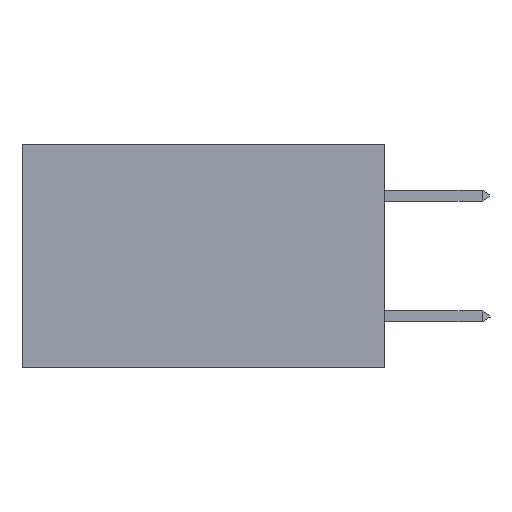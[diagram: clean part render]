
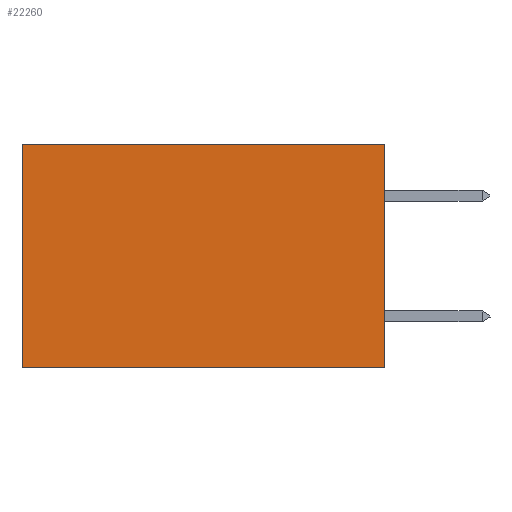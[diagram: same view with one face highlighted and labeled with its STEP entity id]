
A CAD part, left-side view. The second image highlights one B-rep face of the part: STEP entity #22260.
In plain terms, the highlighted planar face has unit normal (-1, 0, 0).
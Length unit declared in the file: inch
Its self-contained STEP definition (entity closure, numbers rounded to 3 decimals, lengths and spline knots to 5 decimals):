
#499 = LINE ( 'NONE', #30578, #22509 ) ;
#1411 = CARTESIAN_POINT ( 'NONE',  ( 0.2875, 0., 0. ) ) ;
#1512 = ORIENTED_EDGE ( 'NONE', *, *, #26970, .F. ) ;
#2909 = CARTESIAN_POINT ( 'NONE',  ( 0.2875, 0., 0. ) ) ;
#3466 = VERTEX_POINT ( 'NONE', #15081 ) ;
#4373 = CARTESIAN_POINT ( 'NONE',  ( 0.2875, 0.6, -0.37 ) ) ;
#5432 = LINE ( 'NONE', #27463, #14908 ) ;
#6847 = EDGE_LOOP ( 'NONE', ( #8869, #7572, #1512, #26331 ) ) ;
#7572 = ORIENTED_EDGE ( 'NONE', *, *, #21735, .F. ) ;
#7997 = VECTOR ( 'NONE', #22997, 39.37008 ) ;
#8869 = ORIENTED_EDGE ( 'NONE', *, *, #30475, .T. ) ;
#10986 = DIRECTION ( 'NONE',  ( 1., 0., 0. ) ) ;
#11207 = CARTESIAN_POINT ( 'NONE',  ( 0.2875, 0.6, 0. ) ) ;
#11342 = DIRECTION ( 'NONE',  ( 0., 0., -1. ) ) ;
#11831 = LINE ( 'NONE', #28019, #7997 ) ;
#14504 = LINE ( 'NONE', #27450, #29020 ) ;
#14908 = VECTOR ( 'NONE', #27703, 39.37008 ) ;
#15081 = CARTESIAN_POINT ( 'NONE',  ( 0.2875, 0., -0.37 ) ) ;
#17165 = FACE_OUTER_BOUND ( 'NONE', #6847, .T. ) ;
#17415 = PLANE ( 'NONE',  #24161 ) ;
#18496 = DIRECTION ( 'NONE',  ( 0., 1., 0. ) ) ;
#18920 = VERTEX_POINT ( 'NONE', #1411 ) ;
#19994 = VERTEX_POINT ( 'NONE', #4373 ) ;
#21735 = EDGE_CURVE ( 'NONE', #3466, #19994, #5432, .T. ) ;
#22260 = ADVANCED_FACE ( 'NONE', ( #17165 ), #17415, .F. ) ;
#22509 = VECTOR ( 'NONE', #11342, 39.37008 ) ;
#22997 = DIRECTION ( 'NONE',  ( 0., 0., -1. ) ) ;
#24161 = AXIS2_PLACEMENT_3D ( 'NONE', #2909, #10986, #30115 ) ;
#24258 = VERTEX_POINT ( 'NONE', #11207 ) ;
#25788 = EDGE_CURVE ( 'NONE', #18920, #24258, #14504, .T. ) ;
#26331 = ORIENTED_EDGE ( 'NONE', *, *, #25788, .T. ) ;
#26970 = EDGE_CURVE ( 'NONE', #18920, #3466, #11831, .T. ) ;
#27450 = CARTESIAN_POINT ( 'NONE',  ( 0.2875, 0., 0. ) ) ;
#27463 = CARTESIAN_POINT ( 'NONE',  ( 0.2875, 0., -0.37 ) ) ;
#27703 = DIRECTION ( 'NONE',  ( 0., 1., 0. ) ) ;
#28019 = CARTESIAN_POINT ( 'NONE',  ( 0.2875, 0., 0. ) ) ;
#29020 = VECTOR ( 'NONE', #18496, 39.37008 ) ;
#30115 = DIRECTION ( 'NONE',  ( 0., 0., -1. ) ) ;
#30475 = EDGE_CURVE ( 'NONE', #24258, #19994, #499, .T. ) ;
#30578 = CARTESIAN_POINT ( 'NONE',  ( 0.2875, 0.6, 0. ) ) ;
